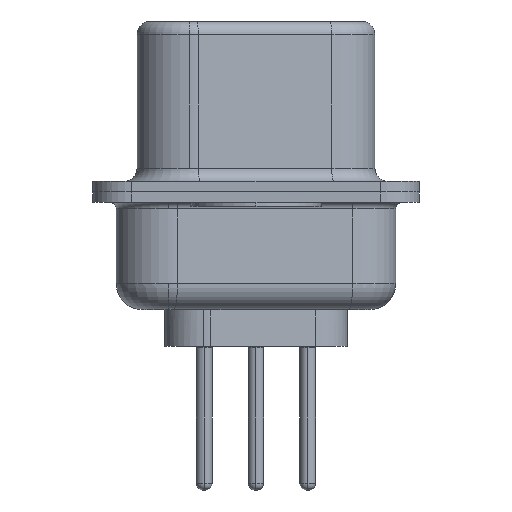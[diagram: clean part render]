
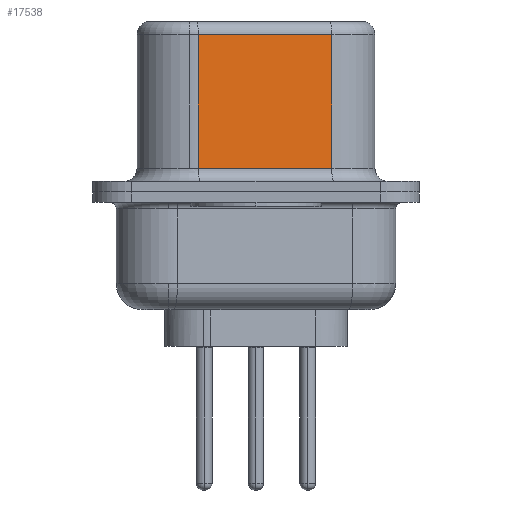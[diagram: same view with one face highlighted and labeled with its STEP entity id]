
A CAD part, left-side view. The second image highlights one B-rep face of the part: STEP entity #17538.
In plain terms, the highlighted planar face has unit normal (-0.985, -0.174, 0).
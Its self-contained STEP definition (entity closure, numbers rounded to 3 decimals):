
#177 = CARTESIAN_POINT ( 'NONE',  ( 4.555, -2.897, 6.52 ) ) ;
#2319 = VERTEX_POINT ( 'NONE', #18188 ) ;
#2832 = ORIENTED_EDGE ( 'NONE', *, *, #14928, .F. ) ;
#2968 = CARTESIAN_POINT ( 'NONE',  ( 4.555, -2.897, 6.02 ) ) ;
#3204 = DIRECTION ( 'NONE',  ( -0.174, 0.985, 0. ) ) ;
#4152 = CARTESIAN_POINT ( 'NONE',  ( 4.555, -2.897, 6.02 ) ) ;
#4240 = EDGE_LOOP ( 'NONE', ( #2832, #7295, #8276, #14140 ) ) ;
#4497 = DIRECTION ( 'NONE',  ( -0.174, 0.985, 0. ) ) ;
#4669 = VERTEX_POINT ( 'NONE', #4152 ) ;
#5769 = LINE ( 'NONE', #9500, #13867 ) ;
#6295 = LINE ( 'NONE', #13355, #10209 ) ;
#7295 = ORIENTED_EDGE ( 'NONE', *, *, #18211, .T. ) ;
#7649 = DIRECTION ( 'NONE',  ( 0., 0., -1. ) ) ;
#8122 = LINE ( 'NONE', #9198, #15172 ) ;
#8245 = AXIS2_PLACEMENT_3D ( 'NONE', #177, #11988, #3204 ) ;
#8276 = ORIENTED_EDGE ( 'NONE', *, *, #10403, .T. ) ;
#9198 = CARTESIAN_POINT ( 'NONE',  ( 4.555, -2.897, 0.9 ) ) ;
#9500 = CARTESIAN_POINT ( 'NONE',  ( 3.655, 2.203, 6.52 ) ) ;
#10209 = VECTOR ( 'NONE', #7649, 1000. ) ;
#10259 = EDGE_CURVE ( 'NONE', #13215, #2319, #8122, .T. ) ;
#10403 = EDGE_CURVE ( 'NONE', #18277, #13215, #5769, .T. ) ;
#10562 = PLANE ( 'NONE',  #8245 ) ;
#10903 = DIRECTION ( 'NONE',  ( 0., 0., -1. ) ) ;
#11882 = VECTOR ( 'NONE', #4497, 1000. ) ;
#11888 = CARTESIAN_POINT ( 'NONE',  ( 3.655, 2.203, 0.9 ) ) ;
#11988 = DIRECTION ( 'NONE',  ( 0.985, 0.174, 0. ) ) ;
#12330 = LINE ( 'NONE', #2968, #11882 ) ;
#13215 = VERTEX_POINT ( 'NONE', #11888 ) ;
#13355 = CARTESIAN_POINT ( 'NONE',  ( 4.555, -2.897, 6.52 ) ) ;
#13867 = VECTOR ( 'NONE', #10903, 1000. ) ;
#14140 = ORIENTED_EDGE ( 'NONE', *, *, #10259, .T. ) ;
#14928 = EDGE_CURVE ( 'NONE', #4669, #2319, #6295, .T. ) ;
#15172 = VECTOR ( 'NONE', #16187, 1000. ) ;
#16112 = CARTESIAN_POINT ( 'NONE',  ( 3.655, 2.203, 6.02 ) ) ;
#16187 = DIRECTION ( 'NONE',  ( 0.174, -0.985, 0. ) ) ;
#17418 = FACE_OUTER_BOUND ( 'NONE', #4240, .T. ) ;
#17538 = ADVANCED_FACE ( 'NONE', ( #17418 ), #10562, .F. ) ;
#18188 = CARTESIAN_POINT ( 'NONE',  ( 4.555, -2.897, 0.9 ) ) ;
#18211 = EDGE_CURVE ( 'NONE', #4669, #18277, #12330, .T. ) ;
#18277 = VERTEX_POINT ( 'NONE', #16112 ) ;
